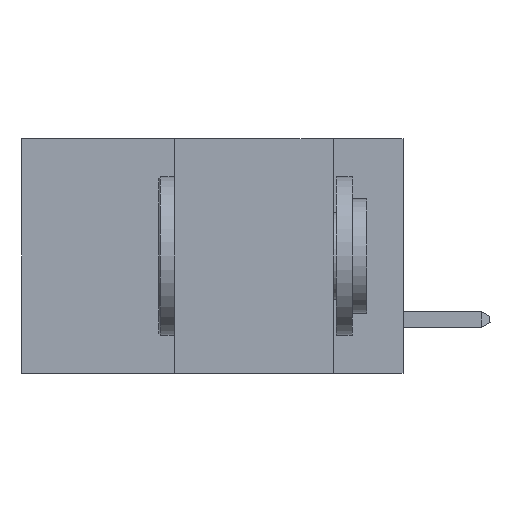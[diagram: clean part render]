
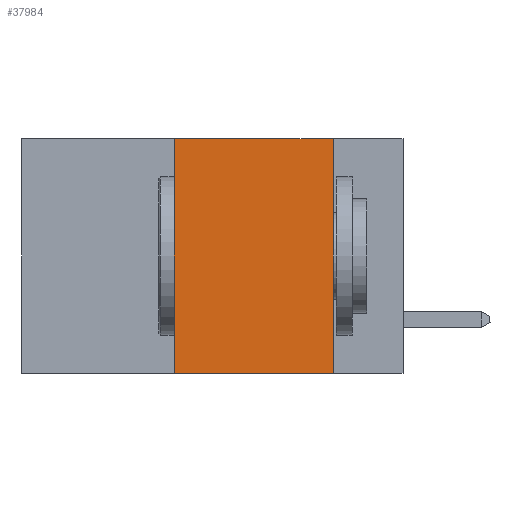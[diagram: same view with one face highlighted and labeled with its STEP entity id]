
A CAD part, left-side view. The second image highlights one B-rep face of the part: STEP entity #37984.
In plain terms, the highlighted planar face has unit normal (-1, 0, 0).
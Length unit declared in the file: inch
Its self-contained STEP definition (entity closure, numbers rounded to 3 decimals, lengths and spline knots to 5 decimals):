
#749 = ORIENTED_EDGE ( 'NONE', *, *, #13630, .T. ) ;
#1044 = VECTOR ( 'NONE', #30867, 39.37008 ) ;
#1288 = EDGE_CURVE ( 'NONE', #26199, #31249, #18345, .T. ) ;
#2150 = CARTESIAN_POINT ( 'NONE',  ( 0., 0.11, 0. ) ) ;
#3104 = ORIENTED_EDGE ( 'NONE', *, *, #20642, .F. ) ;
#3427 = EDGE_CURVE ( 'NONE', #17958, #26199, #38047, .T. ) ;
#5220 = CARTESIAN_POINT ( 'NONE',  ( 0., 0.11, -0.37 ) ) ;
#7139 = CARTESIAN_POINT ( 'NONE',  ( 0., 0.6, 0. ) ) ;
#8126 = EDGE_LOOP ( 'NONE', ( #31122, #26570, #3104, #749 ) ) ;
#8429 = DIRECTION ( 'NONE',  ( 0., 0., -1. ) ) ;
#10222 = VECTOR ( 'NONE', #38713, 39.37008 ) ;
#11662 = VECTOR ( 'NONE', #40721, 39.37008 ) ;
#12320 = CARTESIAN_POINT ( 'NONE',  ( 0., 0.36, -0.37 ) ) ;
#13106 = FACE_OUTER_BOUND ( 'NONE', #8126, .T. ) ;
#13630 = EDGE_CURVE ( 'NONE', #18536, #31249, #22691, .T. ) ;
#14168 = AXIS2_PLACEMENT_3D ( 'NONE', #31033, #16826, #8429 ) ;
#16042 = VECTOR ( 'NONE', #34462, 39.37008 ) ;
#16071 = CARTESIAN_POINT ( 'NONE',  ( 0., 0.6, -0.37 ) ) ;
#16826 = DIRECTION ( 'NONE',  ( 1., 0., 0. ) ) ;
#17958 = VERTEX_POINT ( 'NONE', #19314 ) ;
#18345 = LINE ( 'NONE', #2150, #11662 ) ;
#18536 = VERTEX_POINT ( 'NONE', #12320 ) ;
#19314 = CARTESIAN_POINT ( 'NONE',  ( 0., 0.36, 0. ) ) ;
#20642 = EDGE_CURVE ( 'NONE', #18536, #17958, #34986, .T. ) ;
#22691 = LINE ( 'NONE', #16071, #16042 ) ;
#22909 = PLANE ( 'NONE',  #14168 ) ;
#24993 = CARTESIAN_POINT ( 'NONE',  ( 0., 0.11, 0. ) ) ;
#26199 = VERTEX_POINT ( 'NONE', #24993 ) ;
#26570 = ORIENTED_EDGE ( 'NONE', *, *, #3427, .F. ) ;
#30867 = DIRECTION ( 'NONE',  ( 0., 0., 1. ) ) ;
#31033 = CARTESIAN_POINT ( 'NONE',  ( 0., 0.6, 0. ) ) ;
#31122 = ORIENTED_EDGE ( 'NONE', *, *, #1288, .F. ) ;
#31249 = VERTEX_POINT ( 'NONE', #5220 ) ;
#34462 = DIRECTION ( 'NONE',  ( 0., -1., 0. ) ) ;
#34986 = LINE ( 'NONE', #41260, #1044 ) ;
#37984 = ADVANCED_FACE ( 'NONE', ( #13106 ), #22909, .F. ) ;
#38047 = LINE ( 'NONE', #7139, #10222 ) ;
#38713 = DIRECTION ( 'NONE',  ( 0., -1., 0. ) ) ;
#40721 = DIRECTION ( 'NONE',  ( 0., 0., -1. ) ) ;
#41260 = CARTESIAN_POINT ( 'NONE',  ( 0., 0.36, 0. ) ) ;
